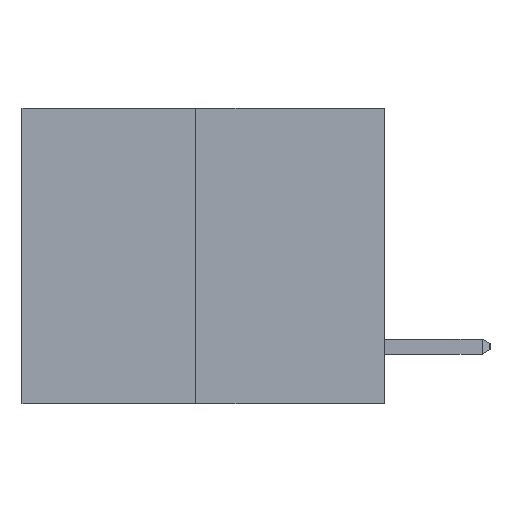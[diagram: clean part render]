
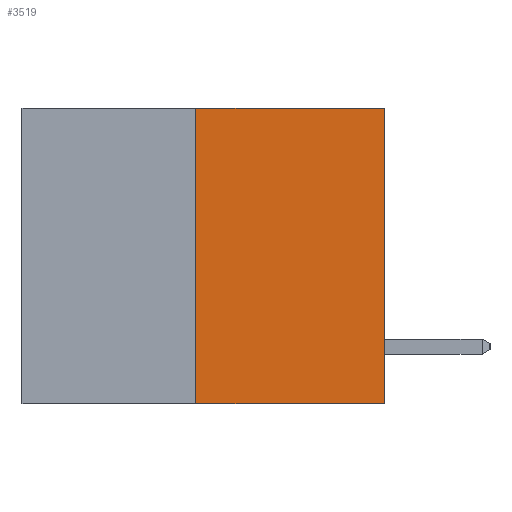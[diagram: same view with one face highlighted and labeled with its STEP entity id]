
A CAD part, left-side view. The second image highlights one B-rep face of the part: STEP entity #3519.
In plain terms, the highlighted planar face has unit normal (-1, 0, 0).
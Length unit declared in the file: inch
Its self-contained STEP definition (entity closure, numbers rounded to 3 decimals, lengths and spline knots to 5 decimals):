
#174 = VECTOR ( 'NONE', #3982, 39.37008 ) ;
#1394 = CARTESIAN_POINT ( 'NONE',  ( 0., 0.6, 0. ) ) ;
#2228 = VERTEX_POINT ( 'NONE', #13719 ) ;
#2385 = DIRECTION ( 'NONE',  ( 0., -1., 0. ) ) ;
#2522 = LINE ( 'NONE', #10500, #8050 ) ;
#3015 = CARTESIAN_POINT ( 'NONE',  ( 0., 0.6, 0. ) ) ;
#3051 = EDGE_CURVE ( 'NONE', #2228, #8032, #3501, .T. ) ;
#3501 = LINE ( 'NONE', #8807, #174 ) ;
#3519 = ADVANCED_FACE ( 'NONE', ( #9844 ), #8940, .F. ) ;
#3893 = AXIS2_PLACEMENT_3D ( 'NONE', #1394, #10376, #5333 ) ;
#3982 = DIRECTION ( 'NONE',  ( 0., 0., 1. ) ) ;
#4450 = EDGE_CURVE ( 'NONE', #14361, #8985, #2522, .T. ) ;
#5074 = ORIENTED_EDGE ( 'NONE', *, *, #12375, .T. ) ;
#5333 = DIRECTION ( 'NONE',  ( 0., 0., -1. ) ) ;
#5344 = DIRECTION ( 'NONE',  ( 0., 0., 1. ) ) ;
#6096 = LINE ( 'NONE', #3015, #8517 ) ;
#7297 = EDGE_LOOP ( 'NONE', ( #8075, #5074, #15665, #13524 ) ) ;
#7605 = CARTESIAN_POINT ( 'NONE',  ( 0., 0.6, -0.49 ) ) ;
#7909 = LINE ( 'NONE', #7605, #10677 ) ;
#8032 = VERTEX_POINT ( 'NONE', #14655 ) ;
#8050 = VECTOR ( 'NONE', #5344, 39.37008 ) ;
#8075 = ORIENTED_EDGE ( 'NONE', *, *, #4450, .F. ) ;
#8517 = VECTOR ( 'NONE', #2385, 39.37008 ) ;
#8807 = CARTESIAN_POINT ( 'NONE',  ( 0., 0., 0. ) ) ;
#8940 = PLANE ( 'NONE',  #3893 ) ;
#8985 = VERTEX_POINT ( 'NONE', #12982 ) ;
#9844 = FACE_OUTER_BOUND ( 'NONE', #7297, .T. ) ;
#10376 = DIRECTION ( 'NONE',  ( 1., 0., 0. ) ) ;
#10500 = CARTESIAN_POINT ( 'NONE',  ( 0., 0.312, -0.49 ) ) ;
#10677 = VECTOR ( 'NONE', #11252, 39.37008 ) ;
#11252 = DIRECTION ( 'NONE',  ( 0., -1., 0. ) ) ;
#11771 = EDGE_CURVE ( 'NONE', #8985, #8032, #6096, .T. ) ;
#12375 = EDGE_CURVE ( 'NONE', #14361, #2228, #7909, .T. ) ;
#12982 = CARTESIAN_POINT ( 'NONE',  ( 0., 0.312, 0. ) ) ;
#13524 = ORIENTED_EDGE ( 'NONE', *, *, #11771, .F. ) ;
#13719 = CARTESIAN_POINT ( 'NONE',  ( 0., 0., -0.49 ) ) ;
#14361 = VERTEX_POINT ( 'NONE', #15114 ) ;
#14655 = CARTESIAN_POINT ( 'NONE',  ( 0., 0., 0. ) ) ;
#15114 = CARTESIAN_POINT ( 'NONE',  ( 0., 0.312, -0.49 ) ) ;
#15665 = ORIENTED_EDGE ( 'NONE', *, *, #3051, .T. ) ;
